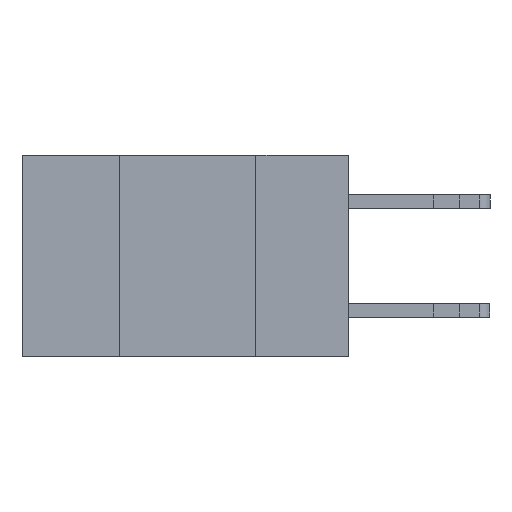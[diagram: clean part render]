
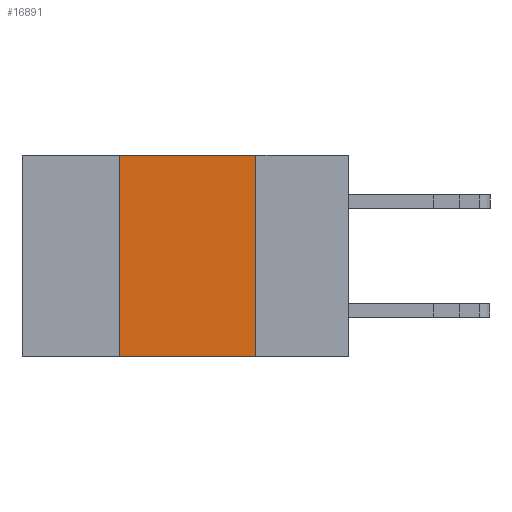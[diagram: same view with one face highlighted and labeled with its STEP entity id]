
A CAD part, left-side view. The second image highlights one B-rep face of the part: STEP entity #16891.
In plain terms, the highlighted planar face has unit normal (-1, 0, 0).
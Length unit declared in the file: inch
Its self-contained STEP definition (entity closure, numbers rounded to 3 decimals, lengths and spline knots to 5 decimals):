
#555 = CARTESIAN_POINT ( 'NONE',  ( 0., 0.42, 0. ) ) ;
#737 = VERTEX_POINT ( 'NONE', #13901 ) ;
#840 = ORIENTED_EDGE ( 'NONE', *, *, #3958, .T. ) ;
#1305 = CARTESIAN_POINT ( 'NONE',  ( 0., 0.6, 0. ) ) ;
#1901 = VECTOR ( 'NONE', #4428, 39.37008 ) ;
#2006 = CARTESIAN_POINT ( 'NONE',  ( 0., 0.6, 0. ) ) ;
#2074 = VECTOR ( 'NONE', #4185, 39.37008 ) ;
#2613 = VERTEX_POINT ( 'NONE', #2926 ) ;
#2630 = EDGE_LOOP ( 'NONE', ( #13548, #3547, #13090, #840 ) ) ;
#2926 = CARTESIAN_POINT ( 'NONE',  ( 0., 0.17, -0.37 ) ) ;
#3454 = DIRECTION ( 'NONE',  ( 0., 0., -1. ) ) ;
#3547 = ORIENTED_EDGE ( 'NONE', *, *, #15240, .F. ) ;
#3958 = EDGE_CURVE ( 'NONE', #737, #2613, #16550, .T. ) ;
#4185 = DIRECTION ( 'NONE',  ( 0., -1., 0. ) ) ;
#4428 = DIRECTION ( 'NONE',  ( 0., -1., 0. ) ) ;
#5382 = EDGE_CURVE ( 'NONE', #15561, #2613, #12763, .T. ) ;
#6323 = CARTESIAN_POINT ( 'NONE',  ( 0., 0.17, 0. ) ) ;
#8126 = VECTOR ( 'NONE', #16167, 39.37008 ) ;
#9108 = DIRECTION ( 'NONE',  ( 0., 0., 1. ) ) ;
#9119 = PLANE ( 'NONE',  #11300 ) ;
#10089 = LINE ( 'NONE', #1305, #2074 ) ;
#10911 = VECTOR ( 'NONE', #9108, 39.37008 ) ;
#11300 = AXIS2_PLACEMENT_3D ( 'NONE', #2006, #11981, #3454 ) ;
#11350 = LINE ( 'NONE', #16151, #10911 ) ;
#11534 = CARTESIAN_POINT ( 'NONE',  ( 0., 0.6, -0.37 ) ) ;
#11930 = EDGE_CURVE ( 'NONE', #737, #14000, #11350, .T. ) ;
#11981 = DIRECTION ( 'NONE',  ( 1., 0., 0. ) ) ;
#12763 = LINE ( 'NONE', #14746, #8126 ) ;
#13090 = ORIENTED_EDGE ( 'NONE', *, *, #11930, .F. ) ;
#13548 = ORIENTED_EDGE ( 'NONE', *, *, #5382, .F. ) ;
#13901 = CARTESIAN_POINT ( 'NONE',  ( 0., 0.42, -0.37 ) ) ;
#14000 = VERTEX_POINT ( 'NONE', #555 ) ;
#14220 = FACE_OUTER_BOUND ( 'NONE', #2630, .T. ) ;
#14746 = CARTESIAN_POINT ( 'NONE',  ( 0., 0.17, 0. ) ) ;
#15240 = EDGE_CURVE ( 'NONE', #14000, #15561, #10089, .T. ) ;
#15561 = VERTEX_POINT ( 'NONE', #6323 ) ;
#16151 = CARTESIAN_POINT ( 'NONE',  ( 0., 0.42, 0. ) ) ;
#16167 = DIRECTION ( 'NONE',  ( 0., 0., -1. ) ) ;
#16550 = LINE ( 'NONE', #11534, #1901 ) ;
#16891 = ADVANCED_FACE ( 'NONE', ( #14220 ), #9119, .F. ) ;
